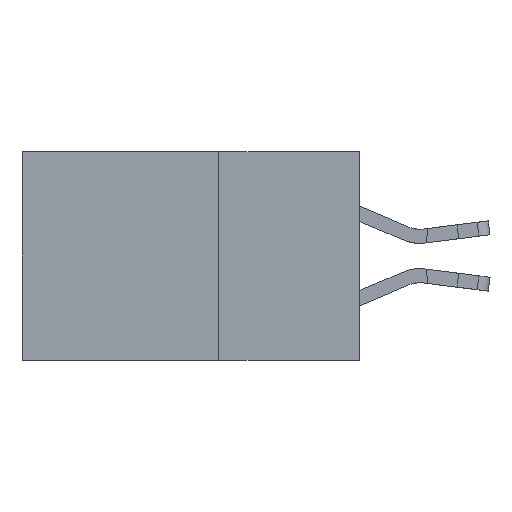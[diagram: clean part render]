
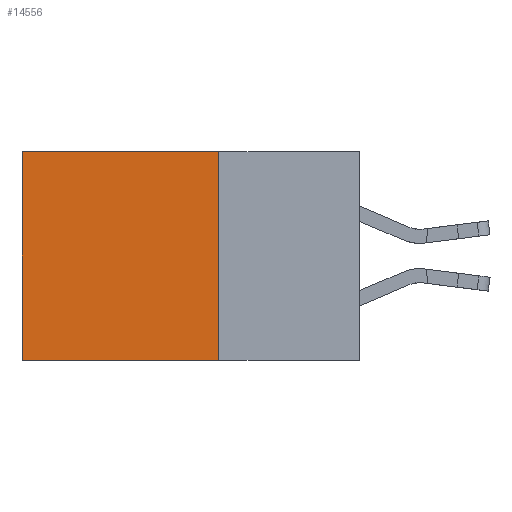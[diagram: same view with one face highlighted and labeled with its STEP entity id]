
A CAD part, left-side view. The second image highlights one B-rep face of the part: STEP entity #14556.
In plain terms, the highlighted planar face has unit normal (-1, 0, 0).
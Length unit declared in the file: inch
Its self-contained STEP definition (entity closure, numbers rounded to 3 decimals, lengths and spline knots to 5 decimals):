
#288 = VECTOR ( 'NONE', #17938, 39.37008 ) ;
#675 = LINE ( 'NONE', #29995, #288 ) ;
#1329 = LINE ( 'NONE', #10156, #30663 ) ;
#1934 = CARTESIAN_POINT ( 'NONE',  ( 0.2875, 0.25, -0.37 ) ) ;
#4566 = CARTESIAN_POINT ( 'NONE',  ( 0.2875, 0.25, 0. ) ) ;
#5650 = DIRECTION ( 'NONE',  ( 0., 0., -1. ) ) ;
#6482 = VERTEX_POINT ( 'NONE', #26215 ) ;
#6654 = EDGE_CURVE ( 'NONE', #21772, #18665, #1329, .T. ) ;
#7061 = AXIS2_PLACEMENT_3D ( 'NONE', #27356, #29333, #5650 ) ;
#7664 = EDGE_CURVE ( 'NONE', #18614, #6482, #27582, .T. ) ;
#10156 = CARTESIAN_POINT ( 'NONE',  ( 0.2875, 0.25, -0.37 ) ) ;
#10739 = PLANE ( 'NONE',  #7061 ) ;
#11317 = ORIENTED_EDGE ( 'NONE', *, *, #7664, .T. ) ;
#12978 = ORIENTED_EDGE ( 'NONE', *, *, #23996, .T. ) ;
#13596 = DIRECTION ( 'NONE',  ( 0., 1., 0. ) ) ;
#14320 = LINE ( 'NONE', #4566, #29947 ) ;
#14556 = ADVANCED_FACE ( 'NONE', ( #28862 ), #10739, .F. ) ;
#14558 = ORIENTED_EDGE ( 'NONE', *, *, #6654, .F. ) ;
#14802 = ORIENTED_EDGE ( 'NONE', *, *, #15235, .F. ) ;
#15235 = EDGE_CURVE ( 'NONE', #18614, #21772, #14320, .T. ) ;
#15905 = CARTESIAN_POINT ( 'NONE',  ( 0.2875, 0.6, -0.37 ) ) ;
#17938 = DIRECTION ( 'NONE',  ( 0., 0., -1. ) ) ;
#18614 = VERTEX_POINT ( 'NONE', #24446 ) ;
#18665 = VERTEX_POINT ( 'NONE', #15905 ) ;
#20665 = CARTESIAN_POINT ( 'NONE',  ( 0.2875, 0.25, 0. ) ) ;
#21772 = VERTEX_POINT ( 'NONE', #1934 ) ;
#22119 = DIRECTION ( 'NONE',  ( 0., 1., 0. ) ) ;
#23996 = EDGE_CURVE ( 'NONE', #6482, #18665, #675, .T. ) ;
#24446 = CARTESIAN_POINT ( 'NONE',  ( 0.2875, 0.25, 0. ) ) ;
#26215 = CARTESIAN_POINT ( 'NONE',  ( 0.2875, 0.6, 0. ) ) ;
#26237 = DIRECTION ( 'NONE',  ( 0., 0., -1. ) ) ;
#27356 = CARTESIAN_POINT ( 'NONE',  ( 0.2875, 0.25, 0. ) ) ;
#27582 = LINE ( 'NONE', #20665, #27931 ) ;
#27931 = VECTOR ( 'NONE', #13596, 39.37008 ) ;
#28022 = EDGE_LOOP ( 'NONE', ( #12978, #14558, #14802, #11317 ) ) ;
#28862 = FACE_OUTER_BOUND ( 'NONE', #28022, .T. ) ;
#29333 = DIRECTION ( 'NONE',  ( 1., 0., 0. ) ) ;
#29947 = VECTOR ( 'NONE', #26237, 39.37008 ) ;
#29995 = CARTESIAN_POINT ( 'NONE',  ( 0.2875, 0.6, 0. ) ) ;
#30663 = VECTOR ( 'NONE', #22119, 39.37008 ) ;
